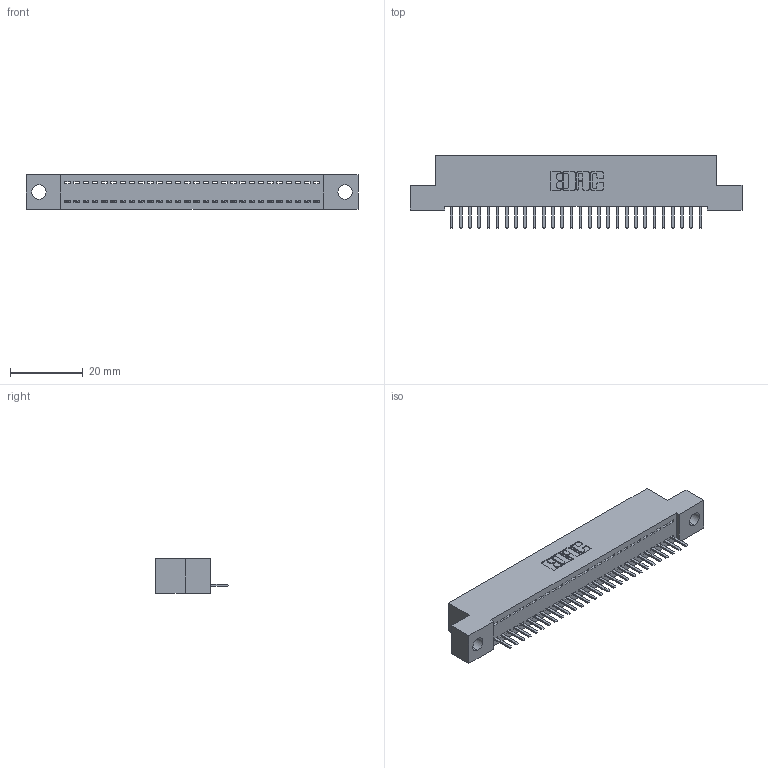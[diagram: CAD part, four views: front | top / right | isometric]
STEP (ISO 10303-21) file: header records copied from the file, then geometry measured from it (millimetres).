
FILE_DESCRIPTION (( 'STEP AP203' ), '1' );
FILE_NAME ('392-028-520-104.STEP', '2018-08-15T20:42:55', ( '' ), ( '' ), 'SwSTEP 2.0', 'SolidWorks 2016', '' );
FILE_SCHEMA (( 'CONFIG_CONTROL_DESIGN' ));
Length unit declared in the file: inch
Products named in the file (3): 342 Part_.156 TH; 345-292-001_345-293-120; 392-028-520-104
Assembly tree (29 placements, depth 2):
  392-028-520-104
    342 Part_.156 TH
    345-292-001_345-293-120  x28
Bounding box: 91.44 x 20.02 x 9.4 mm (x, y, z)
Volume: 7798.3 mm3; surface area: 10751.3 mm2
Topology: 29 solids, 29 shells, 1846 faces, 5451 edges, 3558 vertices
Faces by surface type: plane 1298, cylinder 548
Entity records: 18913 total; most frequent: CARTESIAN_POINT 3282, ORIENTED_EDGE 3234, DIRECTION 2785, EDGE_CURVE 1617, VECTOR 1485, LINE 1485, VERTEX_POINT 1074, AXIS2_PLACEMENT_3D 650
